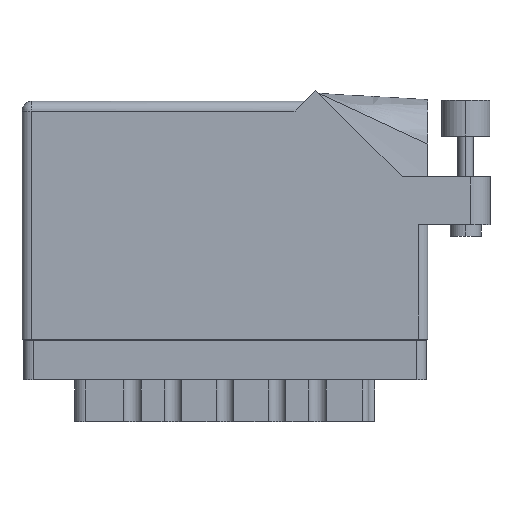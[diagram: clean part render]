
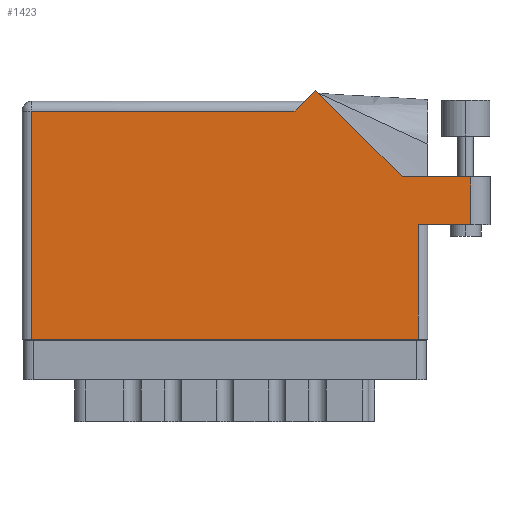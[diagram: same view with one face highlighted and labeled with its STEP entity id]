
A CAD part, front view. The second image highlights one B-rep face of the part: STEP entity #1423.
In plain terms, the highlighted face is planar.
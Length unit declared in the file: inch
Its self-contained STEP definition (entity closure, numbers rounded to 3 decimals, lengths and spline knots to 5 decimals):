
#875 = LINE ( 'NONE', #5388, #13685 ) ;
#1423 = ADVANCED_FACE ( 'NONE', ( #41727 ), #11155, .F. ) ;
#1446 = ORIENTED_EDGE ( 'NONE', *, *, #3807, .T. ) ;
#1808 = DIRECTION ( 'NONE',  ( 1., 0., 0. ) ) ;
#2019 = EDGE_LOOP ( 'NONE', ( #20051, #30809, #24369, #23075, #1446, #25124, #34118, #14755, #11011 ) ) ;
#2600 = VERTEX_POINT ( 'NONE', #18672 ) ;
#2699 = CARTESIAN_POINT ( 'NONE',  ( 1.757, 1.468, 0. ) ) ;
#2911 = DIRECTION ( 'NONE',  ( 0., 1., 0. ) ) ;
#3807 = EDGE_CURVE ( 'NONE', #35595, #27070, #47870, .T. ) ;
#4104 = CARTESIAN_POINT ( 'NONE',  ( 2.612, 0.737, 0. ) ) ;
#5018 = VERTEX_POINT ( 'NONE', #42361 ) ;
#5388 = CARTESIAN_POINT ( 'NONE',  ( 0., 1.468, 0. ) ) ;
#5911 = DIRECTION ( 'NONE',  ( 0., -1., 0. ) ) ;
#6392 = VERTEX_POINT ( 'NONE', #28793 ) ;
#6650 = CARTESIAN_POINT ( 'NONE',  ( 2.887, 0.737, 0. ) ) ;
#7749 = VERTEX_POINT ( 'NONE', #44605 ) ;
#9669 = CARTESIAN_POINT ( 'NONE',  ( 0.062, 0., 0. ) ) ;
#10437 = CARTESIAN_POINT ( 'NONE',  ( 2.55, 0.737, 0. ) ) ;
#11011 = ORIENTED_EDGE ( 'NONE', *, *, #37376, .T. ) ;
#11155 = PLANE ( 'NONE',  #20964 ) ;
#11634 = EDGE_CURVE ( 'NONE', #27070, #5018, #875, .T. ) ;
#11864 = DIRECTION ( 'NONE',  ( -1., 0., 0. ) ) ;
#13685 = VECTOR ( 'NONE', #30953, 39.37008 ) ;
#14755 = ORIENTED_EDGE ( 'NONE', *, *, #38270, .T. ) ;
#15402 = CARTESIAN_POINT ( 'NONE',  ( 0., 1.53, 0. ) ) ;
#16981 = VERTEX_POINT ( 'NONE', #6650 ) ;
#18380 = CARTESIAN_POINT ( 'NONE',  ( 3.012, 1.044, 0. ) ) ;
#18672 = CARTESIAN_POINT ( 'NONE',  ( 2.55, 0., 0. ) ) ;
#19162 = DIRECTION ( 'NONE',  ( 0., 0., -1. ) ) ;
#19377 = DIRECTION ( 'NONE',  ( 1., 0., 0. ) ) ;
#19516 = CARTESIAN_POINT ( 'NONE',  ( 2.44642, 1.044, 0. ) ) ;
#20051 = ORIENTED_EDGE ( 'NONE', *, *, #34555, .T. ) ;
#20964 = AXIS2_PLACEMENT_3D ( 'NONE', #15402, #19162, #26420 ) ;
#21247 = VECTOR ( 'NONE', #19377, 39.37008 ) ;
#21574 = CARTESIAN_POINT ( 'NONE',  ( 0., 0., 0. ) ) ;
#22953 = VECTOR ( 'NONE', #2911, 39.37008 ) ;
#23018 = DIRECTION ( 'NONE',  ( -0.707, 0.707, 0. ) ) ;
#23075 = ORIENTED_EDGE ( 'NONE', *, *, #36603, .T. ) ;
#24275 = LINE ( 'NONE', #39574, #42553 ) ;
#24369 = ORIENTED_EDGE ( 'NONE', *, *, #39165, .T. ) ;
#25124 = ORIENTED_EDGE ( 'NONE', *, *, #11634, .T. ) ;
#25212 = LINE ( 'NONE', #10437, #22953 ) ;
#26309 = VECTOR ( 'NONE', #11864, 39.37008 ) ;
#26420 = DIRECTION ( 'NONE',  ( -1., 0., 0. ) ) ;
#27070 = VERTEX_POINT ( 'NONE', #2699 ) ;
#28114 = LINE ( 'NONE', #4104, #21247 ) ;
#28793 = CARTESIAN_POINT ( 'NONE',  ( 2.55, 0.737, 0. ) ) ;
#30809 = ORIENTED_EDGE ( 'NONE', *, *, #48633, .T. ) ;
#30953 = DIRECTION ( 'NONE',  ( -1., 0., 0. ) ) ;
#30995 = VERTEX_POINT ( 'NONE', #38619 ) ;
#31804 = VECTOR ( 'NONE', #1808, 39.37008 ) ;
#33183 = CARTESIAN_POINT ( 'NONE',  ( 0.062, 0., 0. ) ) ;
#33274 = VECTOR ( 'NONE', #23018, 39.37008 ) ;
#33653 = CARTESIAN_POINT ( 'NONE',  ( 1.88971, 1.60071, 0. ) ) ;
#34118 = ORIENTED_EDGE ( 'NONE', *, *, #41551, .T. ) ;
#34555 = EDGE_CURVE ( 'NONE', #6392, #16981, #28114, .T. ) ;
#35595 = VERTEX_POINT ( 'NONE', #33653 ) ;
#35672 = VECTOR ( 'NONE', #5911, 39.37008 ) ;
#36120 = LINE ( 'NONE', #21574, #31804 ) ;
#36603 = EDGE_CURVE ( 'NONE', #30995, #35595, #42084, .T. ) ;
#37376 = EDGE_CURVE ( 'NONE', #2600, #6392, #25212, .T. ) ;
#37960 = VECTOR ( 'NONE', #47118, 39.37008 ) ;
#38270 = EDGE_CURVE ( 'NONE', #46164, #2600, #36120, .T. ) ;
#38619 = CARTESIAN_POINT ( 'NONE',  ( 2.44642, 1.044, 0. ) ) ;
#39165 = EDGE_CURVE ( 'NONE', #7749, #30995, #48974, .T. ) ;
#39574 = CARTESIAN_POINT ( 'NONE',  ( 2.887, 1.044, 0. ) ) ;
#40488 = LINE ( 'NONE', #9669, #35672 ) ;
#41551 = EDGE_CURVE ( 'NONE', #5018, #46164, #40488, .T. ) ;
#41727 = FACE_OUTER_BOUND ( 'NONE', #2019, .T. ) ;
#42084 = LINE ( 'NONE', #19516, #33274 ) ;
#42361 = CARTESIAN_POINT ( 'NONE',  ( 0.062, 1.468, 0. ) ) ;
#42553 = VECTOR ( 'NONE', #44089, 39.37008 ) ;
#43602 = CARTESIAN_POINT ( 'NONE',  ( 1.819, 1.53, 0. ) ) ;
#44089 = DIRECTION ( 'NONE',  ( 0., 1., 0. ) ) ;
#44605 = CARTESIAN_POINT ( 'NONE',  ( 2.887, 1.044, 0. ) ) ;
#46164 = VERTEX_POINT ( 'NONE', #33183 ) ;
#47118 = DIRECTION ( 'NONE',  ( -0.707, -0.707, 0. ) ) ;
#47870 = LINE ( 'NONE', #43602, #37960 ) ;
#48633 = EDGE_CURVE ( 'NONE', #16981, #7749, #24275, .T. ) ;
#48974 = LINE ( 'NONE', #18380, #26309 ) ;
